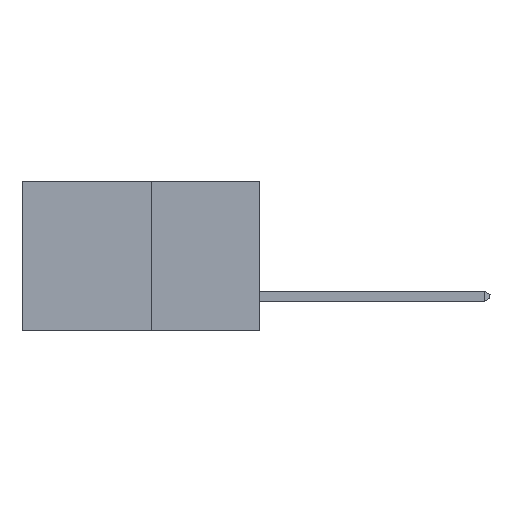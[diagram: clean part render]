
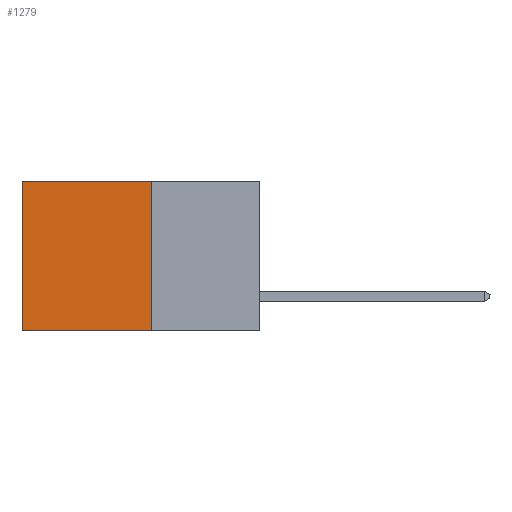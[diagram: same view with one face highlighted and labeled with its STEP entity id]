
A CAD part, left-side view. The second image highlights one B-rep face of the part: STEP entity #1279.
In plain terms, the highlighted planar face has unit normal (-1, 0, 0).
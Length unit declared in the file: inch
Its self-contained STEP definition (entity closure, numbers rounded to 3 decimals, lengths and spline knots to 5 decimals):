
#29 = ORIENTED_EDGE ( 'NONE', *, *, #5801, .F. ) ;
#988 = LINE ( 'NONE', #7129, #7244 ) ;
#1279 = ADVANCED_FACE ( 'NONE', ( #2138 ), #3766, .F. ) ;
#1459 = VECTOR ( 'NONE', #4014, 39.37008 ) ;
#1845 = DIRECTION ( 'NONE',  ( 0., 1., 0. ) ) ;
#1865 = CARTESIAN_POINT ( 'NONE',  ( 0.277, 0.27, 0. ) ) ;
#1909 = AXIS2_PLACEMENT_3D ( 'NONE', #2811, #1970, #6265 ) ;
#1970 = DIRECTION ( 'NONE',  ( 1., 0., 0. ) ) ;
#2138 = FACE_OUTER_BOUND ( 'NONE', #4921, .T. ) ;
#2466 = ORIENTED_EDGE ( 'NONE', *, *, #2944, .F. ) ;
#2650 = VERTEX_POINT ( 'NONE', #2907 ) ;
#2811 = CARTESIAN_POINT ( 'NONE',  ( 0.277, 0.27, -0.37 ) ) ;
#2907 = CARTESIAN_POINT ( 'NONE',  ( 0.277, 0.59, -0.37 ) ) ;
#2944 = EDGE_CURVE ( 'NONE', #4025, #2650, #5879, .T. ) ;
#3087 = LINE ( 'NONE', #4135, #1459 ) ;
#3232 = VERTEX_POINT ( 'NONE', #3533 ) ;
#3533 = CARTESIAN_POINT ( 'NONE',  ( 0.277, 0.59, 0. ) ) ;
#3766 = PLANE ( 'NONE',  #1909 ) ;
#3791 = ORIENTED_EDGE ( 'NONE', *, *, #5659, .T. ) ;
#4004 = CARTESIAN_POINT ( 'NONE',  ( 0.277, 0.27, -0.37 ) ) ;
#4014 = DIRECTION ( 'NONE',  ( 0., 0., -1. ) ) ;
#4025 = VERTEX_POINT ( 'NONE', #4004 ) ;
#4125 = VECTOR ( 'NONE', #1845, 39.37008 ) ;
#4135 = CARTESIAN_POINT ( 'NONE',  ( 0.277, 0.27, -0.37 ) ) ;
#4246 = LINE ( 'NONE', #5811, #7594 ) ;
#4802 = EDGE_CURVE ( 'NONE', #3232, #2650, #988, .T. ) ;
#4921 = EDGE_LOOP ( 'NONE', ( #5160, #2466, #29, #3791 ) ) ;
#5160 = ORIENTED_EDGE ( 'NONE', *, *, #4802, .T. ) ;
#5659 = EDGE_CURVE ( 'NONE', #6975, #3232, #4246, .T. ) ;
#5801 = EDGE_CURVE ( 'NONE', #6975, #4025, #3087, .T. ) ;
#5803 = DIRECTION ( 'NONE',  ( 0., 1., 0. ) ) ;
#5811 = CARTESIAN_POINT ( 'NONE',  ( 0.277, 0.27, 0. ) ) ;
#5879 = LINE ( 'NONE', #6980, #4125 ) ;
#6265 = DIRECTION ( 'NONE',  ( 0., 0., -1. ) ) ;
#6971 = DIRECTION ( 'NONE',  ( 0., 0., -1. ) ) ;
#6975 = VERTEX_POINT ( 'NONE', #1865 ) ;
#6980 = CARTESIAN_POINT ( 'NONE',  ( 0.277, 0.27, -0.37 ) ) ;
#7129 = CARTESIAN_POINT ( 'NONE',  ( 0.277, 0.59, -0.37 ) ) ;
#7244 = VECTOR ( 'NONE', #6971, 39.37008 ) ;
#7594 = VECTOR ( 'NONE', #5803, 39.37008 ) ;
